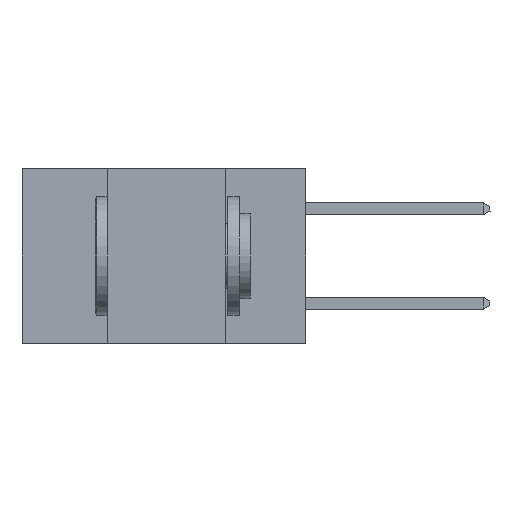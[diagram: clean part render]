
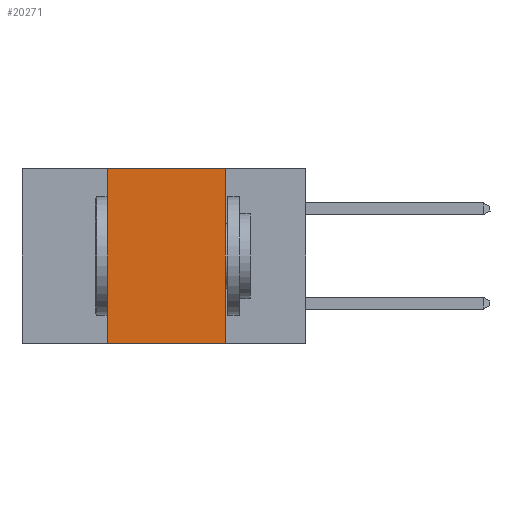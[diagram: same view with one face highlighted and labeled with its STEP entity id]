
A CAD part, left-side view. The second image highlights one B-rep face of the part: STEP entity #20271.
In plain terms, the highlighted planar face has unit normal (-1, 0, 0).
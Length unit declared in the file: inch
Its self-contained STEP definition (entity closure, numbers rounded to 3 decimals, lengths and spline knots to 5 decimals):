
#931 = DIRECTION ( 'NONE',  ( 1., 0., 0. ) ) ;
#1034 = CARTESIAN_POINT ( 'NONE',  ( 0., 0.6, 0. ) ) ;
#1120 = CARTESIAN_POINT ( 'NONE',  ( 0., 0.17, -0.37 ) ) ;
#2039 = EDGE_LOOP ( 'NONE', ( #18644, #10122, #19642, #18729 ) ) ;
#5661 = AXIS2_PLACEMENT_3D ( 'NONE', #1034, #931, #15299 ) ;
#10122 = ORIENTED_EDGE ( 'NONE', *, *, #15825, .F. ) ;
#11775 = EDGE_CURVE ( 'NONE', #29364, #25613, #18492, .T. ) ;
#12874 = DIRECTION ( 'NONE',  ( 0., 0., -1. ) ) ;
#13010 = CARTESIAN_POINT ( 'NONE',  ( 0., 0.17, 0. ) ) ;
#13918 = FACE_OUTER_BOUND ( 'NONE', #2039, .T. ) ;
#15285 = VECTOR ( 'NONE', #30170, 39.37008 ) ;
#15299 = DIRECTION ( 'NONE',  ( 0., 0., -1. ) ) ;
#15654 = LINE ( 'NONE', #17929, #15285 ) ;
#15825 = EDGE_CURVE ( 'NONE', #25613, #31431, #15654, .T. ) ;
#15972 = VECTOR ( 'NONE', #17440, 39.37008 ) ;
#16695 = PLANE ( 'NONE',  #5661 ) ;
#16942 = LINE ( 'NONE', #25275, #24532 ) ;
#17440 = DIRECTION ( 'NONE',  ( 0., -1., 0. ) ) ;
#17929 = CARTESIAN_POINT ( 'NONE',  ( 0., 0.6, 0. ) ) ;
#18492 = LINE ( 'NONE', #22237, #26846 ) ;
#18644 = ORIENTED_EDGE ( 'NONE', *, *, #24025, .F. ) ;
#18729 = ORIENTED_EDGE ( 'NONE', *, *, #29144, .T. ) ;
#19642 = ORIENTED_EDGE ( 'NONE', *, *, #11775, .F. ) ;
#20271 = ADVANCED_FACE ( 'NONE', ( #13918 ), #16695, .F. ) ;
#22237 = CARTESIAN_POINT ( 'NONE',  ( 0., 0.42, 0. ) ) ;
#22884 = CARTESIAN_POINT ( 'NONE',  ( 0., 0.42, 0. ) ) ;
#22943 = VERTEX_POINT ( 'NONE', #1120 ) ;
#24025 = EDGE_CURVE ( 'NONE', #31431, #22943, #16942, .T. ) ;
#24135 = CARTESIAN_POINT ( 'NONE',  ( 0., 0.42, -0.37 ) ) ;
#24532 = VECTOR ( 'NONE', #12874, 39.37008 ) ;
#24688 = DIRECTION ( 'NONE',  ( 0., 0., 1. ) ) ;
#25275 = CARTESIAN_POINT ( 'NONE',  ( 0., 0.17, 0. ) ) ;
#25613 = VERTEX_POINT ( 'NONE', #22884 ) ;
#26846 = VECTOR ( 'NONE', #24688, 39.37008 ) ;
#29144 = EDGE_CURVE ( 'NONE', #29364, #22943, #30856, .T. ) ;
#29266 = CARTESIAN_POINT ( 'NONE',  ( 0., 0.6, -0.37 ) ) ;
#29364 = VERTEX_POINT ( 'NONE', #24135 ) ;
#30170 = DIRECTION ( 'NONE',  ( 0., -1., 0. ) ) ;
#30856 = LINE ( 'NONE', #29266, #15972 ) ;
#31431 = VERTEX_POINT ( 'NONE', #13010 ) ;
